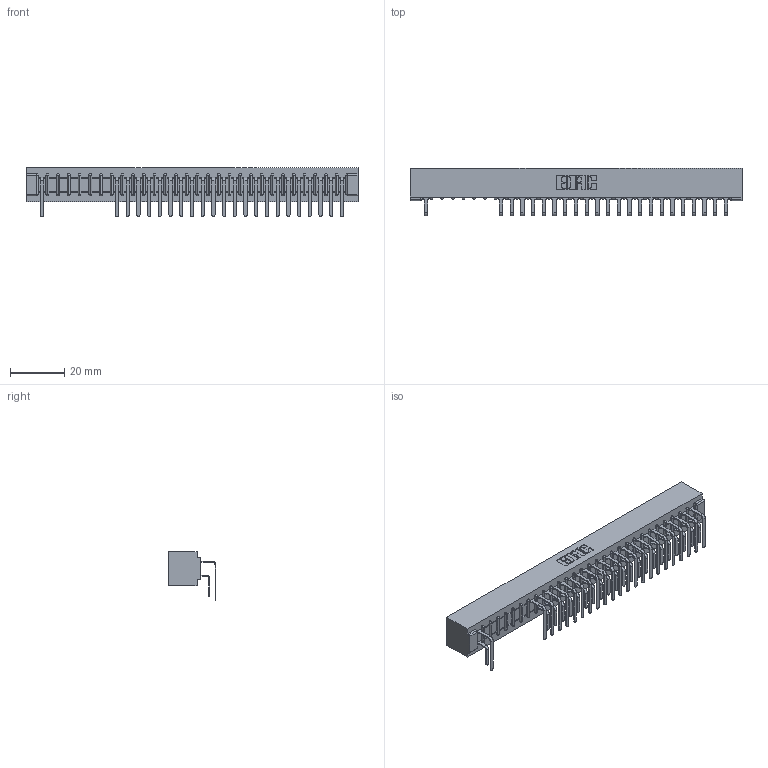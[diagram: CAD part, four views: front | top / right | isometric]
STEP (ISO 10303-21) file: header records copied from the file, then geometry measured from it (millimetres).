
FILE_DESCRIPTION (( 'STEP AP203' ), '1' );
FILE_NAME ('307-058-559-201.STEP', '2018-08-06T07:57:14', ( '' ), ( '' ), 'SwSTEP 2.0', 'SolidWorks 2016', '' );
FILE_SCHEMA (( 'CONFIG_CONTROL_DESIGN' ));
Length unit declared in the file: inch
Products named in the file (4): 307 Part_No Mounting Lugs; 307-290-001_558 559 - 1 (Single); 307-290-001_559 - 2 (Single); 307-058-559-201
Assembly tree (46 placements, depth 2):
  307-058-559-201
    307 Part_No Mounting Lugs
    307-290-001_558 559 - 1 (Single)  x22
    307-290-001_559 - 2 (Single)  x23
Bounding box: 122.78 x 17.69 x 18.07 mm (x, y, z)
Volume: 13544.8 mm3; surface area: 16693.2 mm2
Topology: 46 solids, 46 shells, 2520 faces, 7105 edges, 4594 vertices
Faces by surface type: plane 1629, cylinder 831, sphere 60
Entity records: 28145 total; most frequent: CARTESIAN_POINT 4662, ORIENTED_EDGE 4630, DIRECTION 4557, EDGE_CURVE 2315, VECTOR 1771, LINE 1771, VERTEX_POINT 1498, AXIS2_PLACEMENT_3D 1393
